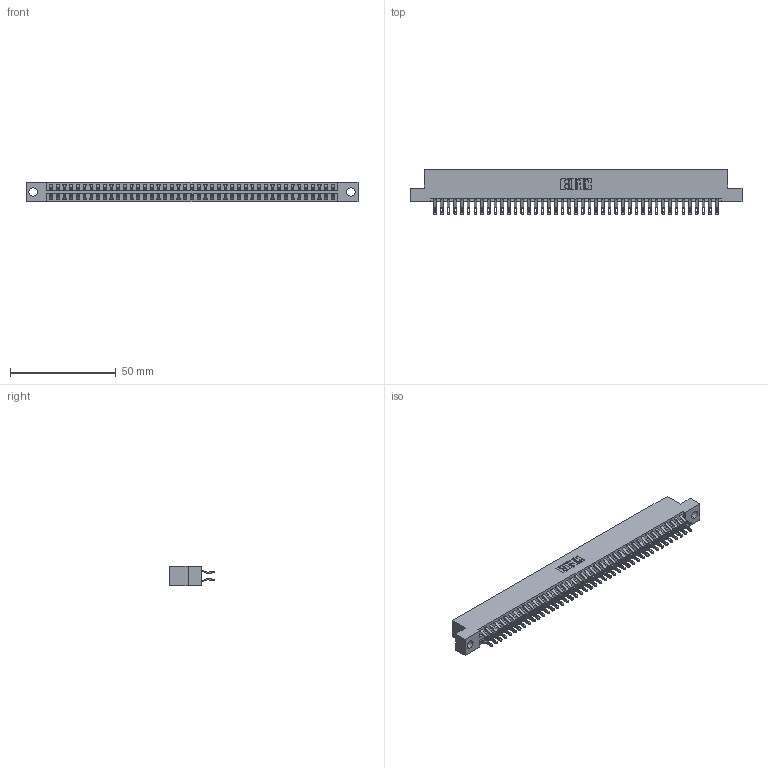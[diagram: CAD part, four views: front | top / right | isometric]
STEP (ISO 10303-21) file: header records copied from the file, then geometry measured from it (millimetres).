
FILE_DESCRIPTION (( 'STEP AP203' ), '1' );
FILE_NAME ('346-086-555-204.STEP', '2022-05-25T22:54:14', ( '' ), ( '' ), 'SwSTEP 2.0', 'SolidWorks 2020', '' );
FILE_SCHEMA (( 'CONFIG_CONTROL_DESIGN' ));
Length unit declared in the file: inch
Products named in the file (3): 346 Part_Flush Mounting Lugs - 0.156 Dia-TH; 345-292-001_555 Tail; 346-086-555-204
Assembly tree (87 placements, depth 2):
  346-086-555-204
    346 Part_Flush Mounting Lugs - 0.156 Dia-TH
    345-292-001_555 Tail  x86
Bounding box: 157.1 x 21.46 x 9.4 mm (x, y, z)
Volume: 15470.4 mm3; surface area: 22017.9 mm2
Topology: 87 solids, 87 shells, 5124 faces, 16103 edges, 10734 vertices
Faces by surface type: plane 2928, cylinder 2196
Entity records: 28673 total; most frequent: CARTESIAN_POINT 4764, ORIENTED_EDGE 4666, DIRECTION 4217, EDGE_CURVE 2333, VECTOR 2009, LINE 2009, VERTEX_POINT 1554, AXIS2_PLACEMENT_3D 1104
